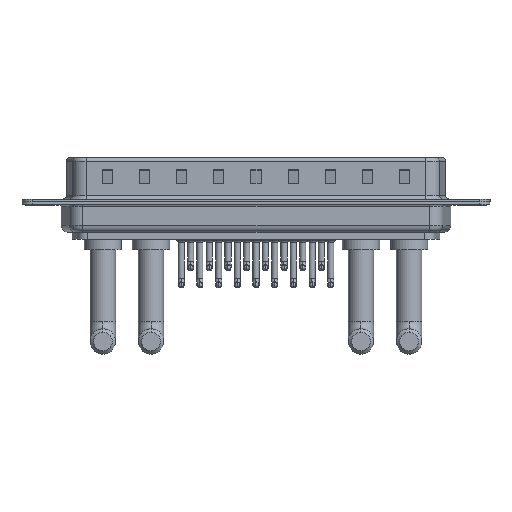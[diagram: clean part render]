
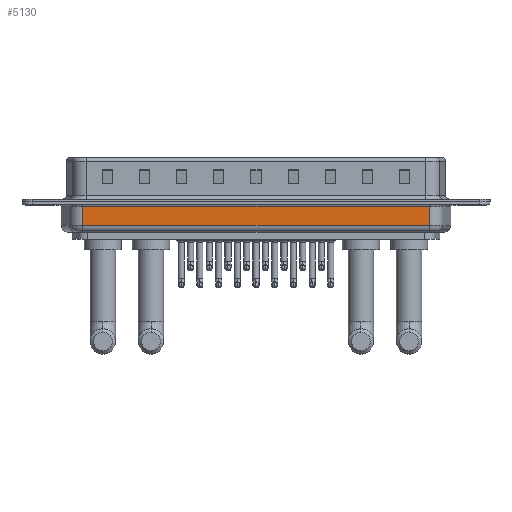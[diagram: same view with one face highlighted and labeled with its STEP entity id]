
A CAD part, front view. The second image highlights one B-rep face of the part: STEP entity #5130.
In plain terms, the highlighted planar face has unit normal (0, -1, 0).
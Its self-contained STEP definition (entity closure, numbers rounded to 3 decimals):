
#721 = AXIS2_PLACEMENT_3D ( 'NONE', #8322, #6663, #12362 ) ;
#2322 = ORIENTED_EDGE ( 'NONE', *, *, #17083, .T. ) ;
#2746 = LINE ( 'NONE', #16603, #4098 ) ;
#3495 = LINE ( 'NONE', #19012, #18412 ) ;
#3762 = CARTESIAN_POINT ( 'NONE',  ( 6.031, -5.35, -0.65 ) ) ;
#4098 = VECTOR ( 'NONE', #10802, 1000. ) ;
#4976 = ORIENTED_EDGE ( 'NONE', *, *, #21866, .T. ) ;
#5130 = ADVANCED_FACE ( 'NONE', ( #10201 ), #12596, .F. ) ;
#5318 = EDGE_CURVE ( 'NONE', #14739, #17169, #20568, .T. ) ;
#6663 = DIRECTION ( 'NONE',  ( 0., 1., 0. ) ) ;
#8322 = CARTESIAN_POINT ( 'NONE',  ( 6.031, -5.35, -4.5 ) ) ;
#8566 = EDGE_CURVE ( 'NONE', #17647, #10579, #2746, .T. ) ;
#9194 = ORIENTED_EDGE ( 'NONE', *, *, #5318, .F. ) ;
#10201 = FACE_OUTER_BOUND ( 'NONE', #20596, .T. ) ;
#10579 = VERTEX_POINT ( 'NONE', #15873 ) ;
#10802 = DIRECTION ( 'NONE',  ( 0., 0., 1. ) ) ;
#12362 = DIRECTION ( 'NONE',  ( -1., 0., 0. ) ) ;
#12596 = PLANE ( 'NONE',  #721 ) ;
#14739 = VERTEX_POINT ( 'NONE', #18232 ) ;
#14875 = DIRECTION ( 'NONE',  ( 0., 0., 1. ) ) ;
#15704 = CARTESIAN_POINT ( 'NONE',  ( 57.469, -5.35, -3.5 ) ) ;
#15862 = CARTESIAN_POINT ( 'NONE',  ( 6.031, -5.35, -0.65 ) ) ;
#15873 = CARTESIAN_POINT ( 'NONE',  ( 57.469, -5.35, -0.65 ) ) ;
#16028 = VECTOR ( 'NONE', #14875, 1000. ) ;
#16297 = VECTOR ( 'NONE', #22720, 1000. ) ;
#16603 = CARTESIAN_POINT ( 'NONE',  ( 57.469, -5.35, -4.5 ) ) ;
#16882 = LINE ( 'NONE', #3762, #16297 ) ;
#17083 = EDGE_CURVE ( 'NONE', #10579, #17169, #16882, .T. ) ;
#17169 = VERTEX_POINT ( 'NONE', #15862 ) ;
#17647 = VERTEX_POINT ( 'NONE', #15704 ) ;
#18232 = CARTESIAN_POINT ( 'NONE',  ( 6.031, -5.35, -3.5 ) ) ;
#18412 = VECTOR ( 'NONE', #18893, 1000. ) ;
#18893 = DIRECTION ( 'NONE',  ( 1., 0., 0. ) ) ;
#19012 = CARTESIAN_POINT ( 'NONE',  ( 6.031, -5.35, -3.5 ) ) ;
#19323 = ORIENTED_EDGE ( 'NONE', *, *, #8566, .T. ) ;
#20568 = LINE ( 'NONE', #24748, #16028 ) ;
#20596 = EDGE_LOOP ( 'NONE', ( #9194, #4976, #19323, #2322 ) ) ;
#21866 = EDGE_CURVE ( 'NONE', #14739, #17647, #3495, .T. ) ;
#22720 = DIRECTION ( 'NONE',  ( -1., 0., 0. ) ) ;
#24748 = CARTESIAN_POINT ( 'NONE',  ( 6.031, -5.35, -4.5 ) ) ;
